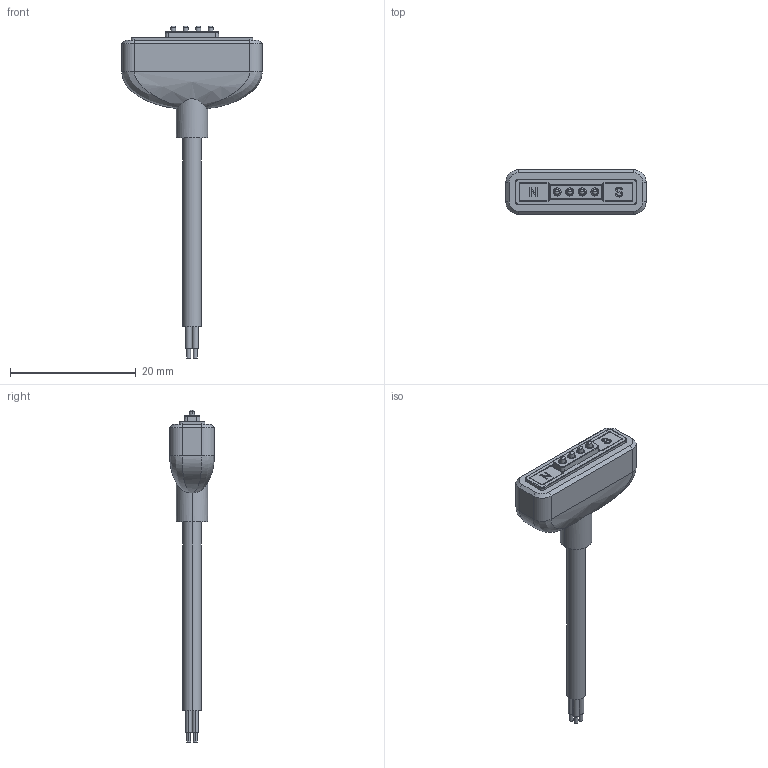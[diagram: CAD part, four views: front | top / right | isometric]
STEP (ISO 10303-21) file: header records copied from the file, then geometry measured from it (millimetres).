
FILE_DESCRIPTION (( 'STEP AP203' ), '1' );
FILE_NAME ('687-J0421051110A.STEP', '2023-02-11T06:13:19', ( '' ), ( '' ), 'SwSTEP 2.0', 'SolidWorks 2020', '' );
FILE_SCHEMA (( 'CONFIG_CONTROL_DESIGN' ));
Length unit declared in the file: millimetre
Products named in the file (1): 687-J0421051110A
Bounding box: 22.3 x 7.1 x 52.8 mm (x, y, z)
Volume: 1376.7 mm3; surface area: 1732.3 mm2
Topology: 1 solids, 4 shells, 302 faces, 708 edges, 448 vertices
Faces by surface type: plane 118, cylinder 106, bspline 38, torus 16, cone 16, sphere 8
Entity records: 12251 total; most frequent: CARTESIAN_POINT 5307, DIRECTION 1421, ORIENTED_EDGE 1416, EDGE_CURVE 708, AXIS2_PLACEMENT_3D 533, VERTEX_POINT 448, LINE 355, VECTOR 355
